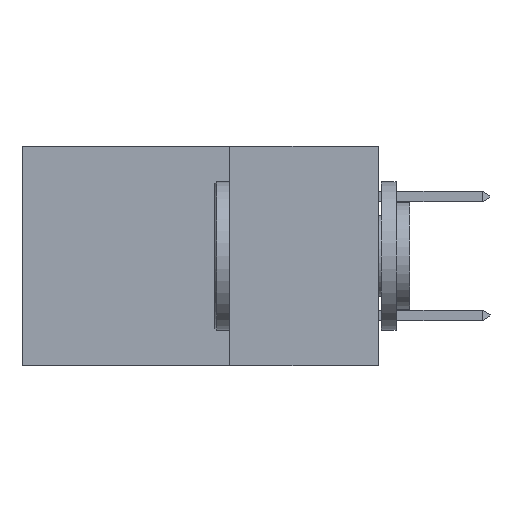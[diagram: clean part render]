
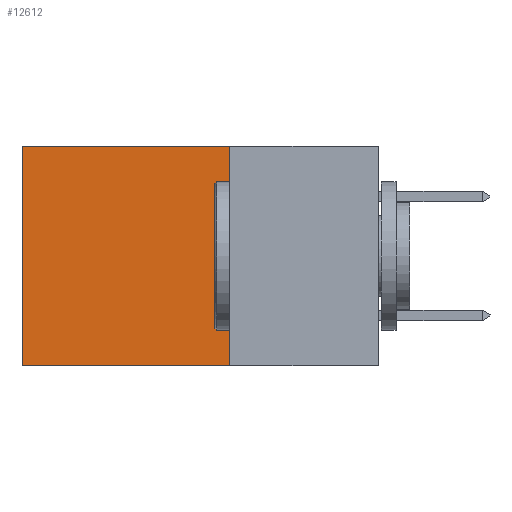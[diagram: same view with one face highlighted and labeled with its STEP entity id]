
A CAD part, left-side view. The second image highlights one B-rep face of the part: STEP entity #12612.
In plain terms, the highlighted planar face has unit normal (-1, 0, 0).
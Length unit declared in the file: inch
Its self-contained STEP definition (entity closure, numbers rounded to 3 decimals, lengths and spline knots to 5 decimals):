
#404 = DIRECTION ( 'NONE',  ( 0., 1., 0. ) ) ;
#633 = EDGE_CURVE ( 'NONE', #3165, #10963, #13808, .T. ) ;
#1119 = DIRECTION ( 'NONE',  ( 0., 0., -1. ) ) ;
#1403 = CARTESIAN_POINT ( 'NONE',  ( 0.298, 0.25, -0.37 ) ) ;
#2457 = CARTESIAN_POINT ( 'NONE',  ( 0.298, 0.6, 0. ) ) ;
#2521 = CARTESIAN_POINT ( 'NONE',  ( 0.298, 0.25, 0. ) ) ;
#2732 = EDGE_CURVE ( 'NONE', #15885, #3144, #6561, .T. ) ;
#2893 = VECTOR ( 'NONE', #404, 39.37008 ) ;
#3144 = VERTEX_POINT ( 'NONE', #11698 ) ;
#3165 = VERTEX_POINT ( 'NONE', #13503 ) ;
#4834 = CARTESIAN_POINT ( 'NONE',  ( 0.298, 0.25, 0. ) ) ;
#5002 = LINE ( 'NONE', #15281, #2893 ) ;
#5528 = DIRECTION ( 'NONE',  ( 0., 1., 0. ) ) ;
#6561 = LINE ( 'NONE', #13193, #10479 ) ;
#6664 = DIRECTION ( 'NONE',  ( 1., 0., 0. ) ) ;
#6858 = DIRECTION ( 'NONE',  ( 0., 0., -1. ) ) ;
#7907 = ORIENTED_EDGE ( 'NONE', *, *, #2732, .T. ) ;
#8701 = ORIENTED_EDGE ( 'NONE', *, *, #633, .F. ) ;
#9390 = AXIS2_PLACEMENT_3D ( 'NONE', #14088, #6664, #6858 ) ;
#9919 = FACE_OUTER_BOUND ( 'NONE', #11210, .T. ) ;
#10479 = VECTOR ( 'NONE', #1119, 39.37008 ) ;
#10963 = VERTEX_POINT ( 'NONE', #1403 ) ;
#11210 = EDGE_LOOP ( 'NONE', ( #7907, #18340, #8701, #15860 ) ) ;
#11698 = CARTESIAN_POINT ( 'NONE',  ( 0.298, 0.6, -0.37 ) ) ;
#12612 = ADVANCED_FACE ( 'NONE', ( #9919 ), #17171, .F. ) ;
#13193 = CARTESIAN_POINT ( 'NONE',  ( 0.298, 0.6, 0. ) ) ;
#13503 = CARTESIAN_POINT ( 'NONE',  ( 0.298, 0.25, 0. ) ) ;
#13808 = LINE ( 'NONE', #4834, #18830 ) ;
#13871 = DIRECTION ( 'NONE',  ( 0., 0., -1. ) ) ;
#13908 = LINE ( 'NONE', #2521, #16201 ) ;
#14088 = CARTESIAN_POINT ( 'NONE',  ( 0.298, 0.25, 0. ) ) ;
#15281 = CARTESIAN_POINT ( 'NONE',  ( 0.298, 0.25, -0.37 ) ) ;
#15860 = ORIENTED_EDGE ( 'NONE', *, *, #16007, .T. ) ;
#15885 = VERTEX_POINT ( 'NONE', #2457 ) ;
#16007 = EDGE_CURVE ( 'NONE', #3165, #15885, #13908, .T. ) ;
#16201 = VECTOR ( 'NONE', #5528, 39.37008 ) ;
#17171 = PLANE ( 'NONE',  #9390 ) ;
#18340 = ORIENTED_EDGE ( 'NONE', *, *, #18581, .F. ) ;
#18581 = EDGE_CURVE ( 'NONE', #10963, #3144, #5002, .T. ) ;
#18830 = VECTOR ( 'NONE', #13871, 39.37008 ) ;
